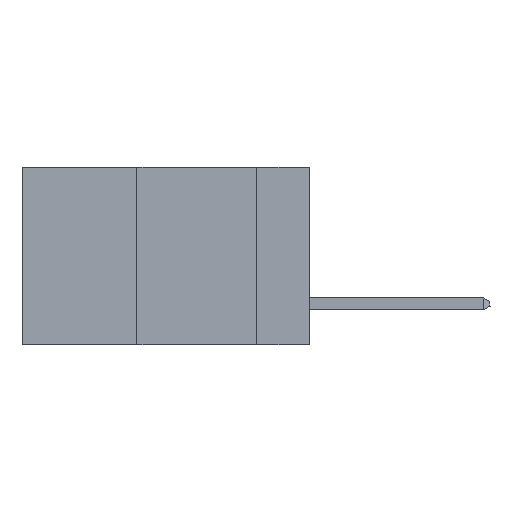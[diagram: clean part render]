
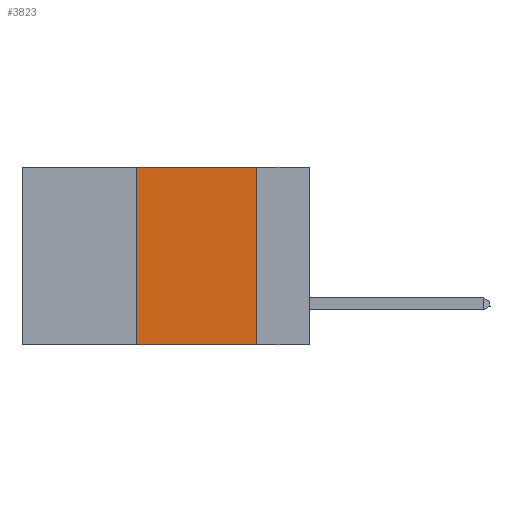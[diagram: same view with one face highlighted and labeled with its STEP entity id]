
A CAD part, left-side view. The second image highlights one B-rep face of the part: STEP entity #3823.
In plain terms, the highlighted planar face has unit normal (-1, 0, 0).
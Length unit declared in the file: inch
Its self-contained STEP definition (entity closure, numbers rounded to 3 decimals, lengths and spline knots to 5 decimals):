
#27 = ORIENTED_EDGE ( 'NONE', *, *, #4052, .F. ) ;
#154 = LINE ( 'NONE', #509, #19218 ) ;
#280 = VERTEX_POINT ( 'NONE', #22534 ) ;
#509 = CARTESIAN_POINT ( 'NONE',  ( 0., 0.36, 0. ) ) ;
#823 = AXIS2_PLACEMENT_3D ( 'NONE', #4602, #17736, #13521 ) ;
#884 = ORIENTED_EDGE ( 'NONE', *, *, #21242, .T. ) ;
#1349 = ORIENTED_EDGE ( 'NONE', *, *, #14640, .F. ) ;
#1536 = FACE_OUTER_BOUND ( 'NONE', #11415, .T. ) ;
#3028 = CARTESIAN_POINT ( 'NONE',  ( 0., 0.11, 0. ) ) ;
#3823 = ADVANCED_FACE ( 'NONE', ( #1536 ), #16425, .F. ) ;
#4030 = DIRECTION ( 'NONE',  ( 0., 0., 1. ) ) ;
#4052 = EDGE_CURVE ( 'NONE', #18598, #8268, #4941, .T. ) ;
#4602 = CARTESIAN_POINT ( 'NONE',  ( 0., 0.6, 0. ) ) ;
#4941 = LINE ( 'NONE', #8849, #20243 ) ;
#5636 = LINE ( 'NONE', #7049, #14426 ) ;
#6739 = CARTESIAN_POINT ( 'NONE',  ( 0., 0.11, 0. ) ) ;
#7049 = CARTESIAN_POINT ( 'NONE',  ( 0., 0.6, -0.37 ) ) ;
#8268 = VERTEX_POINT ( 'NONE', #3028 ) ;
#8664 = LINE ( 'NONE', #6739, #10383 ) ;
#8849 = CARTESIAN_POINT ( 'NONE',  ( 0., 0.6, 0. ) ) ;
#8928 = DIRECTION ( 'NONE',  ( 0., -1., 0. ) ) ;
#10383 = VECTOR ( 'NONE', #19767, 39.37008 ) ;
#11415 = EDGE_LOOP ( 'NONE', ( #1349, #27, #22855, #884 ) ) ;
#12217 = CARTESIAN_POINT ( 'NONE',  ( 0., 0.36, 0. ) ) ;
#13521 = DIRECTION ( 'NONE',  ( 0., 0., -1. ) ) ;
#14426 = VECTOR ( 'NONE', #8928, 39.37008 ) ;
#14640 = EDGE_CURVE ( 'NONE', #8268, #17647, #8664, .T. ) ;
#16425 = PLANE ( 'NONE',  #823 ) ;
#16568 = CARTESIAN_POINT ( 'NONE',  ( 0., 0.11, -0.37 ) ) ;
#17633 = DIRECTION ( 'NONE',  ( 0., -1., 0. ) ) ;
#17647 = VERTEX_POINT ( 'NONE', #16568 ) ;
#17736 = DIRECTION ( 'NONE',  ( 1., 0., 0. ) ) ;
#18598 = VERTEX_POINT ( 'NONE', #12217 ) ;
#19033 = EDGE_CURVE ( 'NONE', #280, #18598, #154, .T. ) ;
#19218 = VECTOR ( 'NONE', #4030, 39.37008 ) ;
#19767 = DIRECTION ( 'NONE',  ( 0., 0., -1. ) ) ;
#20243 = VECTOR ( 'NONE', #17633, 39.37008 ) ;
#21242 = EDGE_CURVE ( 'NONE', #280, #17647, #5636, .T. ) ;
#22534 = CARTESIAN_POINT ( 'NONE',  ( 0., 0.36, -0.37 ) ) ;
#22855 = ORIENTED_EDGE ( 'NONE', *, *, #19033, .F. ) ;
